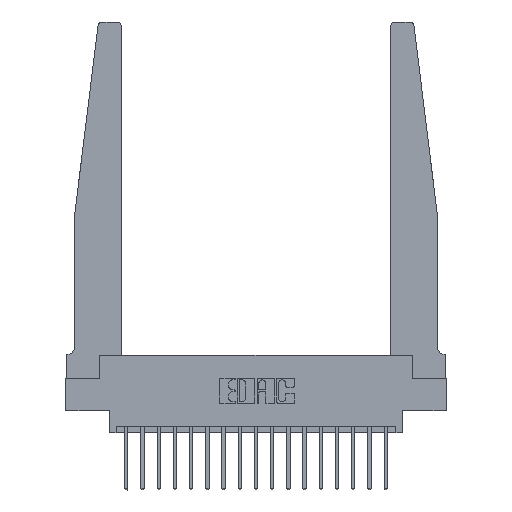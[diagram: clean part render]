
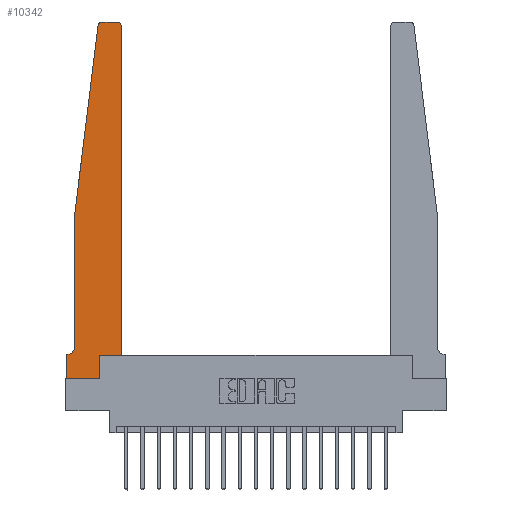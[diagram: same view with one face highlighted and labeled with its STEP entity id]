
A CAD part, top view. The second image highlights one B-rep face of the part: STEP entity #10342.
In plain terms, the highlighted planar face has unit normal (0, 0, 1).
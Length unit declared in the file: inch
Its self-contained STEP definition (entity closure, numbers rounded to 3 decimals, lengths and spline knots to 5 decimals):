
#33 = CARTESIAN_POINT ( 'NONE',  ( 0.2605, 0.18, 0.37 ) ) ;
#150 = EDGE_CURVE ( 'NONE', #518, #17680, #1173, .T. ) ;
#518 = VERTEX_POINT ( 'NONE', #7965 ) ;
#807 = LINE ( 'NONE', #12408, #8433 ) ;
#911 = CARTESIAN_POINT ( 'NONE',  ( 0.27653, 2.72, 0.37 ) ) ;
#1069 = VECTOR ( 'NONE', #15754, 39.37008 ) ;
#1173 = CIRCLE ( 'NONE', #1297, 0.05 ) ;
#1209 = LINE ( 'NONE', #9657, #12783 ) ;
#1297 = AXIS2_PLACEMENT_3D ( 'NONE', #2990, #2966, #15732 ) ;
#1358 = LINE ( 'NONE', #4920, #5937 ) ;
#1543 = LINE ( 'NONE', #9773, #1069 ) ;
#1664 = CARTESIAN_POINT ( 'NONE',  ( 0.2605, 0., 0.37 ) ) ;
#1702 = CARTESIAN_POINT ( 'NONE',  ( 0.425, 2.72, 0.37 ) ) ;
#2458 = DIRECTION ( 'NONE',  ( 1., 0., 0. ) ) ;
#2508 = CARTESIAN_POINT ( 'NONE',  ( 0.425, 0.18, 0.37 ) ) ;
#2532 = DIRECTION ( 'NONE',  ( 0., 0., 1. ) ) ;
#2966 = DIRECTION ( 'NONE',  ( 0., 0., -1. ) ) ;
#2990 = CARTESIAN_POINT ( 'NONE',  ( 0.015, 0.2375, 0.37 ) ) ;
#3891 = ORIENTED_EDGE ( 'NONE', *, *, #4942, .T. ) ;
#3979 = VECTOR ( 'NONE', #12695, 39.37008 ) ;
#4201 = ORIENTED_EDGE ( 'NONE', *, *, #8431, .T. ) ;
#4216 = CARTESIAN_POINT ( 'NONE',  ( 0.2605, 0.18, 0.37 ) ) ;
#4299 = CARTESIAN_POINT ( 'NONE',  ( 0., 0.1875, 0.37 ) ) ;
#4454 = FACE_OUTER_BOUND ( 'NONE', #14744, .T. ) ;
#4641 = DIRECTION ( 'NONE',  ( 0., 1., 0. ) ) ;
#4920 = CARTESIAN_POINT ( 'NONE',  ( 0., 0., 0.37 ) ) ;
#4942 = EDGE_CURVE ( 'NONE', #13224, #10843, #807, .T. ) ;
#4977 = VECTOR ( 'NONE', #11824, 39.37008 ) ;
#5453 = LINE ( 'NONE', #10328, #4977 ) ;
#5937 = VECTOR ( 'NONE', #15358, 39.37008 ) ;
#6646 = CARTESIAN_POINT ( 'NONE',  ( 0.065, 0.1875, 0.37 ) ) ;
#6716 = CARTESIAN_POINT ( 'NONE',  ( 0.25, 2.75, 0.37 ) ) ;
#6930 = ORIENTED_EDGE ( 'NONE', *, *, #17493, .T. ) ;
#7174 = VERTEX_POINT ( 'NONE', #1664 ) ;
#7229 = ORIENTED_EDGE ( 'NONE', *, *, #11405, .T. ) ;
#7417 = ORIENTED_EDGE ( 'NONE', *, *, #18942, .T. ) ;
#7724 = VECTOR ( 'NONE', #12640, 39.37008 ) ;
#7838 = VERTEX_POINT ( 'NONE', #1702 ) ;
#7855 = VECTOR ( 'NONE', #4641, 39.37008 ) ;
#7965 = CARTESIAN_POINT ( 'NONE',  ( 0.065, 0.2375, 0.37 ) ) ;
#8094 = CIRCLE ( 'NONE', #11131, 0.03 ) ;
#8308 = LINE ( 'NONE', #33, #7855 ) ;
#8431 = EDGE_CURVE ( 'NONE', #7174, #13224, #8308, .T. ) ;
#8433 = VECTOR ( 'NONE', #13909, 39.37008 ) ;
#8599 = CARTESIAN_POINT ( 'NONE',  ( 0.395, 2.72, 0.37 ) ) ;
#8613 = VERTEX_POINT ( 'NONE', #17314 ) ;
#9347 = EDGE_CURVE ( 'NONE', #8613, #7174, #5453, .T. ) ;
#9657 = CARTESIAN_POINT ( 'NONE',  ( 0.065, 1.25, 0.37 ) ) ;
#9696 = ORIENTED_EDGE ( 'NONE', *, *, #9347, .T. ) ;
#9773 = CARTESIAN_POINT ( 'NONE',  ( 0.425, 0.18, 0.37 ) ) ;
#9910 = VERTEX_POINT ( 'NONE', #19382 ) ;
#10080 = PLANE ( 'NONE',  #13562 ) ;
#10092 = DIRECTION ( 'NONE',  ( 1., 0., 0. ) ) ;
#10328 = CARTESIAN_POINT ( 'NONE',  ( 0., 0., 0.37 ) ) ;
#10342 = ADVANCED_FACE ( 'NONE', ( #4454 ), #10080, .T. ) ;
#10485 = ORIENTED_EDGE ( 'NONE', *, *, #18208, .T. ) ;
#10843 = VERTEX_POINT ( 'NONE', #2508 ) ;
#11123 = DIRECTION ( 'NONE',  ( -0.122, -0.992, 0. ) ) ;
#11131 = AXIS2_PLACEMENT_3D ( 'NONE', #911, #11493, #2458 ) ;
#11405 = EDGE_CURVE ( 'NONE', #9910, #518, #12443, .T. ) ;
#11439 = CARTESIAN_POINT ( 'NONE',  ( 0.24675, 2.72367, 0.37 ) ) ;
#11493 = DIRECTION ( 'NONE',  ( 0., 0., 1. ) ) ;
#11562 = CARTESIAN_POINT ( 'NONE',  ( 0., 0.1875, 0.37 ) ) ;
#11824 = DIRECTION ( 'NONE',  ( 1., 0., 0. ) ) ;
#12030 = EDGE_CURVE ( 'NONE', #10843, #7838, #1543, .T. ) ;
#12088 = VERTEX_POINT ( 'NONE', #11439 ) ;
#12131 = LINE ( 'NONE', #6716, #7724 ) ;
#12408 = CARTESIAN_POINT ( 'NONE',  ( 0.425, 0.18, 0.37 ) ) ;
#12443 = LINE ( 'NONE', #17069, #3979 ) ;
#12573 = VECTOR ( 'NONE', #15540, 39.37008 ) ;
#12640 = DIRECTION ( 'NONE',  ( -1., 0., 0. ) ) ;
#12695 = DIRECTION ( 'NONE',  ( 0., -1., 0. ) ) ;
#12751 = VERTEX_POINT ( 'NONE', #4299 ) ;
#12783 = VECTOR ( 'NONE', #11123, 39.37008 ) ;
#12904 = ORIENTED_EDGE ( 'NONE', *, *, #150, .T. ) ;
#13048 = DIRECTION ( 'NONE',  ( 1., 0., 0. ) ) ;
#13224 = VERTEX_POINT ( 'NONE', #4216 ) ;
#13300 = CARTESIAN_POINT ( 'NONE',  ( 0.395, 2.75, 0.37 ) ) ;
#13562 = AXIS2_PLACEMENT_3D ( 'NONE', #11562, #2532, #13048 ) ;
#13909 = DIRECTION ( 'NONE',  ( 1., 0., 0. ) ) ;
#14215 = ORIENTED_EDGE ( 'NONE', *, *, #12030, .T. ) ;
#14311 = EDGE_CURVE ( 'NONE', #17970, #19037, #12131, .T. ) ;
#14408 = CIRCLE ( 'NONE', #16852, 0.03 ) ;
#14744 = EDGE_LOOP ( 'NONE', ( #17080, #16041, #7417, #7229, #12904, #10485, #6930, #9696, #4201, #3891, #14215, #16199 ) ) ;
#15358 = DIRECTION ( 'NONE',  ( 0., -1., 0. ) ) ;
#15540 = DIRECTION ( 'NONE',  ( -1., 0., 0. ) ) ;
#15700 = CARTESIAN_POINT ( 'NONE',  ( 0.27653, 2.75, 0.37 ) ) ;
#15732 = DIRECTION ( 'NONE',  ( -1., 0., 0. ) ) ;
#15754 = DIRECTION ( 'NONE',  ( 0., 1., 0. ) ) ;
#16041 = ORIENTED_EDGE ( 'NONE', *, *, #17089, .T. ) ;
#16199 = ORIENTED_EDGE ( 'NONE', *, *, #19074, .T. ) ;
#16852 = AXIS2_PLACEMENT_3D ( 'NONE', #8599, #18917, #10092 ) ;
#16956 = LINE ( 'NONE', #6646, #12573 ) ;
#17069 = CARTESIAN_POINT ( 'NONE',  ( 0.065, 1.25, 0.37 ) ) ;
#17080 = ORIENTED_EDGE ( 'NONE', *, *, #14311, .T. ) ;
#17089 = EDGE_CURVE ( 'NONE', #19037, #12088, #8094, .T. ) ;
#17314 = CARTESIAN_POINT ( 'NONE',  ( 0., 0., 0.37 ) ) ;
#17493 = EDGE_CURVE ( 'NONE', #12751, #8613, #1358, .T. ) ;
#17680 = VERTEX_POINT ( 'NONE', #18614 ) ;
#17970 = VERTEX_POINT ( 'NONE', #13300 ) ;
#18208 = EDGE_CURVE ( 'NONE', #17680, #12751, #16956, .T. ) ;
#18614 = CARTESIAN_POINT ( 'NONE',  ( 0.015, 0.1875, 0.37 ) ) ;
#18917 = DIRECTION ( 'NONE',  ( 0., 0., 1. ) ) ;
#18942 = EDGE_CURVE ( 'NONE', #12088, #9910, #1209, .T. ) ;
#19037 = VERTEX_POINT ( 'NONE', #15700 ) ;
#19074 = EDGE_CURVE ( 'NONE', #7838, #17970, #14408, .T. ) ;
#19382 = CARTESIAN_POINT ( 'NONE',  ( 0.065, 1.25, 0.37 ) ) ;
